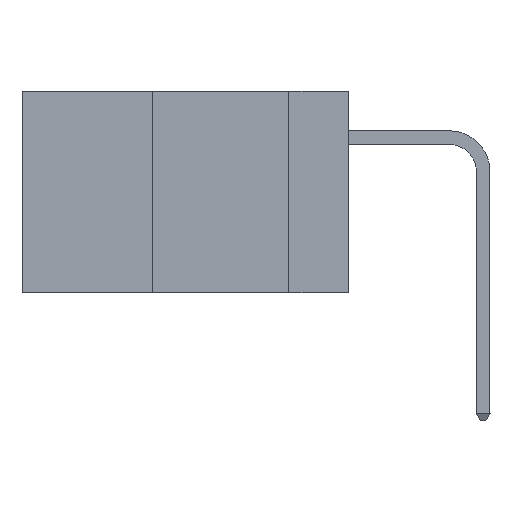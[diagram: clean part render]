
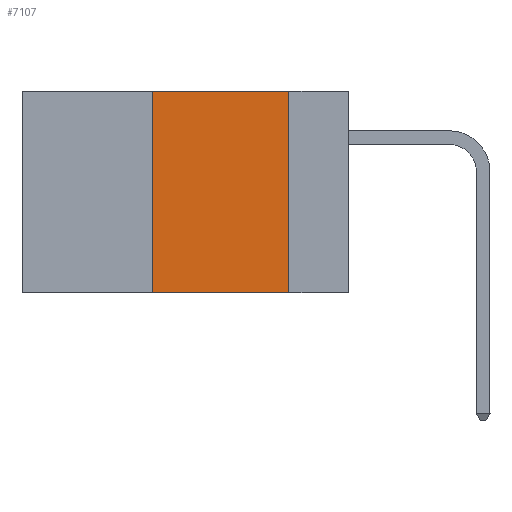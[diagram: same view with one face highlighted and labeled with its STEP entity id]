
A CAD part, left-side view. The second image highlights one B-rep face of the part: STEP entity #7107.
In plain terms, the highlighted planar face has unit normal (-1, 0, 0).
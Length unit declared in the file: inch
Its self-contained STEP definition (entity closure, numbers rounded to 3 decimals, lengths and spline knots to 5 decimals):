
#157 = DIRECTION ( 'NONE',  ( 0., -1., 0. ) ) ;
#1003 = LINE ( 'NONE', #6350, #8387 ) ;
#1037 = ORIENTED_EDGE ( 'NONE', *, *, #7965, .F. ) ;
#1575 = VECTOR ( 'NONE', #9877, 39.37008 ) ;
#2278 = CARTESIAN_POINT ( 'NONE',  ( 0., 0.36, -0.37 ) ) ;
#2340 = CARTESIAN_POINT ( 'NONE',  ( 0., 0.6, -0.37 ) ) ;
#2749 = VERTEX_POINT ( 'NONE', #6613 ) ;
#2933 = CARTESIAN_POINT ( 'NONE',  ( 0., 0.36, 0. ) ) ;
#3151 = DIRECTION ( 'NONE',  ( 0., -1., 0. ) ) ;
#3174 = PLANE ( 'NONE',  #3224 ) ;
#3224 = AXIS2_PLACEMENT_3D ( 'NONE', #7825, #9189, #3778 ) ;
#3447 = EDGE_CURVE ( 'NONE', #5017, #4444, #9270, .T. ) ;
#3495 = CARTESIAN_POINT ( 'NONE',  ( 0., 0.36, 0. ) ) ;
#3578 = DIRECTION ( 'NONE',  ( 0., 0., -1. ) ) ;
#3778 = DIRECTION ( 'NONE',  ( 0., 0., -1. ) ) ;
#4444 = VERTEX_POINT ( 'NONE', #5888 ) ;
#5017 = VERTEX_POINT ( 'NONE', #2278 ) ;
#5798 = ORIENTED_EDGE ( 'NONE', *, *, #3447, .T. ) ;
#5865 = EDGE_CURVE ( 'NONE', #2749, #4444, #7624, .T. ) ;
#5888 = CARTESIAN_POINT ( 'NONE',  ( 0., 0.11, -0.37 ) ) ;
#6350 = CARTESIAN_POINT ( 'NONE',  ( 0., 0.6, 0. ) ) ;
#6613 = CARTESIAN_POINT ( 'NONE',  ( 0., 0.11, 0. ) ) ;
#6962 = FACE_OUTER_BOUND ( 'NONE', #8930, .T. ) ;
#7044 = VECTOR ( 'NONE', #3151, 39.37008 ) ;
#7107 = ADVANCED_FACE ( 'NONE', ( #6962 ), #3174, .F. ) ;
#7238 = VECTOR ( 'NONE', #3578, 39.37008 ) ;
#7438 = ORIENTED_EDGE ( 'NONE', *, *, #7654, .F. ) ;
#7624 = LINE ( 'NONE', #9854, #7238 ) ;
#7654 = EDGE_CURVE ( 'NONE', #8261, #2749, #1003, .T. ) ;
#7825 = CARTESIAN_POINT ( 'NONE',  ( 0., 0.6, 0. ) ) ;
#7965 = EDGE_CURVE ( 'NONE', #5017, #8261, #9974, .T. ) ;
#8261 = VERTEX_POINT ( 'NONE', #3495 ) ;
#8387 = VECTOR ( 'NONE', #157, 39.37008 ) ;
#8930 = EDGE_LOOP ( 'NONE', ( #9518, #7438, #1037, #5798 ) ) ;
#9189 = DIRECTION ( 'NONE',  ( 1., 0., 0. ) ) ;
#9270 = LINE ( 'NONE', #2340, #7044 ) ;
#9518 = ORIENTED_EDGE ( 'NONE', *, *, #5865, .F. ) ;
#9854 = CARTESIAN_POINT ( 'NONE',  ( 0., 0.11, 0. ) ) ;
#9877 = DIRECTION ( 'NONE',  ( 0., 0., 1. ) ) ;
#9974 = LINE ( 'NONE', #2933, #1575 ) ;
